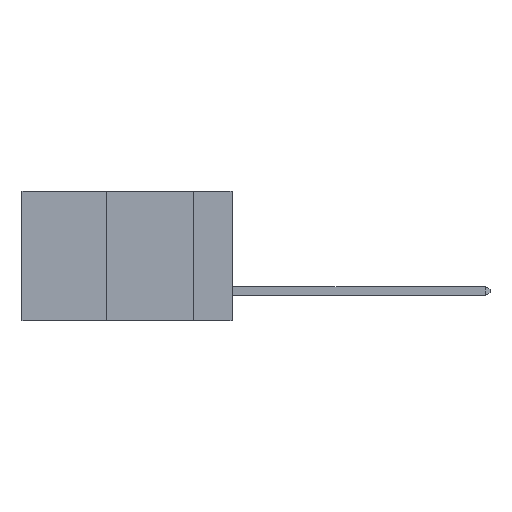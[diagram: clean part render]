
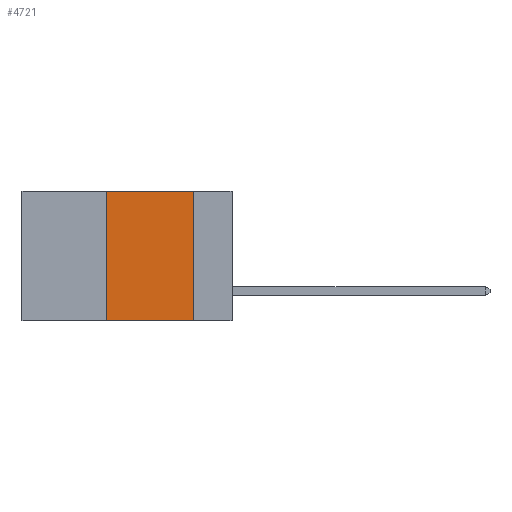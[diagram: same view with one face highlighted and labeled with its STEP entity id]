
A CAD part, left-side view. The second image highlights one B-rep face of the part: STEP entity #4721.
In plain terms, the highlighted planar face has unit normal (-1, 0, 0).
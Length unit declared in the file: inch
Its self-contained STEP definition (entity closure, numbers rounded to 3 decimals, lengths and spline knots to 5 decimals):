
#52 = LINE ( 'NONE', #7855, #3269 ) ;
#504 = DIRECTION ( 'NONE',  ( 0., 0., 1. ) ) ;
#625 = DIRECTION ( 'NONE',  ( 0., 0., -1. ) ) ;
#684 = DIRECTION ( 'NONE',  ( 0., 0., -1. ) ) ;
#699 = DIRECTION ( 'NONE',  ( 1., 0., 0. ) ) ;
#738 = CARTESIAN_POINT ( 'NONE',  ( 0., 0.6, 0. ) ) ;
#818 = PLANE ( 'NONE',  #13669 ) ;
#1213 = CARTESIAN_POINT ( 'NONE',  ( 0., 0.6, -0.37 ) ) ;
#1847 = VERTEX_POINT ( 'NONE', #12146 ) ;
#2946 = VERTEX_POINT ( 'NONE', #14097 ) ;
#3269 = VECTOR ( 'NONE', #5502, 39.37008 ) ;
#4428 = ORIENTED_EDGE ( 'NONE', *, *, #12923, .T. ) ;
#4566 = VECTOR ( 'NONE', #504, 39.37008 ) ;
#4721 = ADVANCED_FACE ( 'NONE', ( #9077 ), #818, .F. ) ;
#5214 = CARTESIAN_POINT ( 'NONE',  ( 0., 0.36, 0. ) ) ;
#5320 = CARTESIAN_POINT ( 'NONE',  ( 0., 0.11, 0. ) ) ;
#5347 = LINE ( 'NONE', #8897, #11087 ) ;
#5502 = DIRECTION ( 'NONE',  ( 0., -1., 0. ) ) ;
#5595 = VERTEX_POINT ( 'NONE', #5320 ) ;
#6567 = LINE ( 'NONE', #1213, #9311 ) ;
#6991 = CARTESIAN_POINT ( 'NONE',  ( 0., 0.36, 0. ) ) ;
#7855 = CARTESIAN_POINT ( 'NONE',  ( 0., 0.6, 0. ) ) ;
#8897 = CARTESIAN_POINT ( 'NONE',  ( 0., 0.11, 0. ) ) ;
#9077 = FACE_OUTER_BOUND ( 'NONE', #10282, .T. ) ;
#9244 = ORIENTED_EDGE ( 'NONE', *, *, #12715, .F. ) ;
#9311 = VECTOR ( 'NONE', #9440, 39.37008 ) ;
#9440 = DIRECTION ( 'NONE',  ( 0., -1., 0. ) ) ;
#10282 = EDGE_LOOP ( 'NONE', ( #11217, #9244, #13427, #4428 ) ) ;
#10288 = EDGE_CURVE ( 'NONE', #5595, #2946, #5347, .T. ) ;
#10719 = LINE ( 'NONE', #5214, #4566 ) ;
#11087 = VECTOR ( 'NONE', #625, 39.37008 ) ;
#11217 = ORIENTED_EDGE ( 'NONE', *, *, #10288, .F. ) ;
#11475 = EDGE_CURVE ( 'NONE', #1847, #12275, #10719, .T. ) ;
#12146 = CARTESIAN_POINT ( 'NONE',  ( 0., 0.36, -0.37 ) ) ;
#12275 = VERTEX_POINT ( 'NONE', #6991 ) ;
#12715 = EDGE_CURVE ( 'NONE', #12275, #5595, #52, .T. ) ;
#12923 = EDGE_CURVE ( 'NONE', #1847, #2946, #6567, .T. ) ;
#13427 = ORIENTED_EDGE ( 'NONE', *, *, #11475, .F. ) ;
#13669 = AXIS2_PLACEMENT_3D ( 'NONE', #738, #699, #684 ) ;
#14097 = CARTESIAN_POINT ( 'NONE',  ( 0., 0.11, -0.37 ) ) ;
